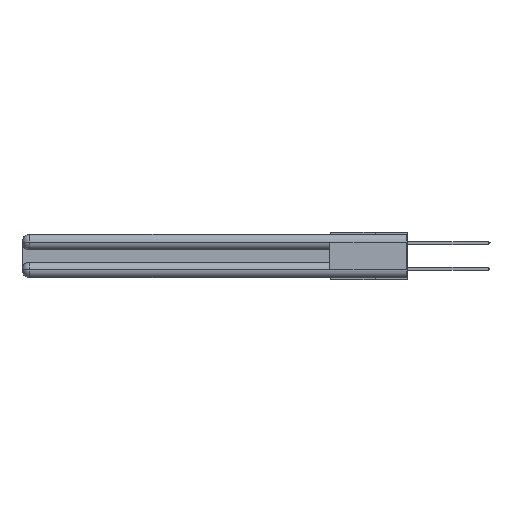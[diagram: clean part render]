
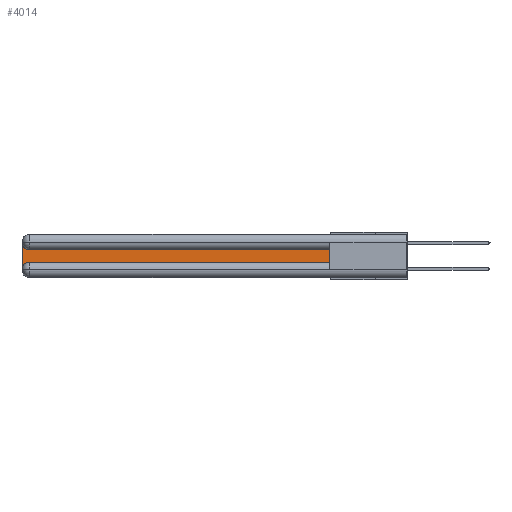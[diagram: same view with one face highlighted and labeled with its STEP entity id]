
A CAD part, left-side view. The second image highlights one B-rep face of the part: STEP entity #4014.
In plain terms, the highlighted planar face has unit normal (-1, 0, 0).
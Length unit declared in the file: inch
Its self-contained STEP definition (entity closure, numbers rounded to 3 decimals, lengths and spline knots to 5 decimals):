
#551 = CARTESIAN_POINT ( 'NONE',  ( 0.075, 2.94, -0.2175 ) ) ;
#625 = ORIENTED_EDGE ( 'NONE', *, *, #5002, .T. ) ;
#1887 = VERTEX_POINT ( 'NONE', #551 ) ;
#3488 = EDGE_CURVE ( 'NONE', #1887, #23557, #19861, .T. ) ;
#3830 = DIRECTION ( 'NONE',  ( 1., 0., 0. ) ) ;
#4014 = ADVANCED_FACE ( 'NONE', ( #20328 ), #22912, .F. ) ;
#4068 = LINE ( 'NONE', #20715, #19769 ) ;
#4902 = CARTESIAN_POINT ( 'NONE',  ( 0.075, 3., -0.0625 ) ) ;
#4953 = LINE ( 'NONE', #11868, #19189 ) ;
#4996 = DIRECTION ( 'NONE',  ( 0., 1., 0. ) ) ;
#5002 = EDGE_CURVE ( 'NONE', #23557, #26543, #8199, .T. ) ;
#5037 = DIRECTION ( 'NONE',  ( 0., 0., -1. ) ) ;
#5369 = EDGE_CURVE ( 'NONE', #26543, #15156, #4953, .T. ) ;
#5631 = EDGE_CURVE ( 'NONE', #15156, #11921, #13880, .T. ) ;
#5760 = CARTESIAN_POINT ( 'NONE',  ( 0.075, 0.6, -0.2175 ) ) ;
#6445 = AXIS2_PLACEMENT_3D ( 'NONE', #13943, #27700, #20835 ) ;
#7575 = VERTEX_POINT ( 'NONE', #12825 ) ;
#7790 = ORIENTED_EDGE ( 'NONE', *, *, #5369, .T. ) ;
#7818 = EDGE_CURVE ( 'NONE', #11921, #7575, #4068, .T. ) ;
#8199 = LINE ( 'NONE', #26370, #19571 ) ;
#9143 = AXIS2_PLACEMENT_3D ( 'NONE', #28378, #3830, #19655 ) ;
#9189 = VECTOR ( 'NONE', #16987, 39.37008 ) ;
#10324 = DIRECTION ( 'NONE',  ( 0., 0., -1. ) ) ;
#11225 = ORIENTED_EDGE ( 'NONE', *, *, #5631, .T. ) ;
#11868 = CARTESIAN_POINT ( 'NONE',  ( 0.075, 0.6, -0.1225 ) ) ;
#11921 = VERTEX_POINT ( 'NONE', #4902 ) ;
#12825 = CARTESIAN_POINT ( 'NONE',  ( 0.075, 3., -0.2775 ) ) ;
#13559 = CARTESIAN_POINT ( 'NONE',  ( 0.075, 0.6, -0.1225 ) ) ;
#13880 = CIRCLE ( 'NONE', #9143, 0.06 ) ;
#13943 = CARTESIAN_POINT ( 'NONE',  ( 0.075, 3., -0.1225 ) ) ;
#14213 = CARTESIAN_POINT ( 'NONE',  ( 0.075, 2.94, -0.1225 ) ) ;
#15156 = VERTEX_POINT ( 'NONE', #14213 ) ;
#15173 = ORIENTED_EDGE ( 'NONE', *, *, #3488, .T. ) ;
#15736 = EDGE_CURVE ( 'NONE', #7575, #1887, #17074, .T. ) ;
#16987 = DIRECTION ( 'NONE',  ( 0., -1., 0. ) ) ;
#17074 = CIRCLE ( 'NONE', #28315, 0.06 ) ;
#17178 = DIRECTION ( 'NONE',  ( 1., 0., 0. ) ) ;
#19189 = VECTOR ( 'NONE', #4996, 39.37008 ) ;
#19571 = VECTOR ( 'NONE', #21680, 39.37008 ) ;
#19655 = DIRECTION ( 'NONE',  ( 0., 0., -1. ) ) ;
#19769 = VECTOR ( 'NONE', #5037, 39.37008 ) ;
#19837 = CARTESIAN_POINT ( 'NONE',  ( 0.075, 0.6, -0.2175 ) ) ;
#19861 = LINE ( 'NONE', #5760, #9189 ) ;
#20328 = FACE_OUTER_BOUND ( 'NONE', #21568, .T. ) ;
#20715 = CARTESIAN_POINT ( 'NONE',  ( 0.075, 3., -0.2175 ) ) ;
#20835 = DIRECTION ( 'NONE',  ( 0., 0., -1. ) ) ;
#21309 = ORIENTED_EDGE ( 'NONE', *, *, #15736, .T. ) ;
#21568 = EDGE_LOOP ( 'NONE', ( #7790, #11225, #25452, #21309, #15173, #625 ) ) ;
#21680 = DIRECTION ( 'NONE',  ( 0., 0., 1. ) ) ;
#21706 = CARTESIAN_POINT ( 'NONE',  ( 0.075, 2.94, -0.2775 ) ) ;
#22912 = PLANE ( 'NONE',  #6445 ) ;
#23557 = VERTEX_POINT ( 'NONE', #19837 ) ;
#25452 = ORIENTED_EDGE ( 'NONE', *, *, #7818, .T. ) ;
#26370 = CARTESIAN_POINT ( 'NONE',  ( 0.075, 0.6, -0.2175 ) ) ;
#26543 = VERTEX_POINT ( 'NONE', #13559 ) ;
#27700 = DIRECTION ( 'NONE',  ( 1., 0., 0. ) ) ;
#28315 = AXIS2_PLACEMENT_3D ( 'NONE', #21706, #17178, #10324 ) ;
#28378 = CARTESIAN_POINT ( 'NONE',  ( 0.075, 2.94, -0.0625 ) ) ;
